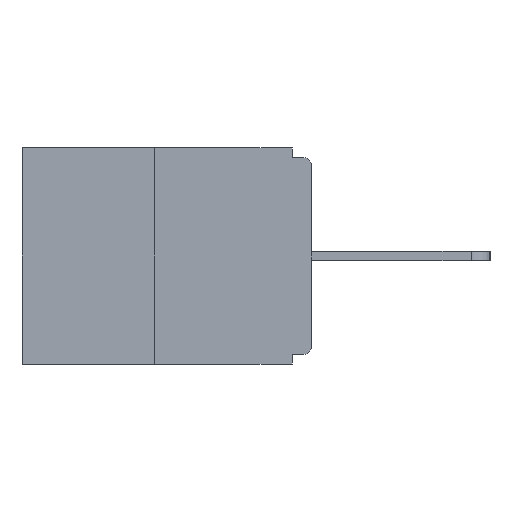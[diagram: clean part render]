
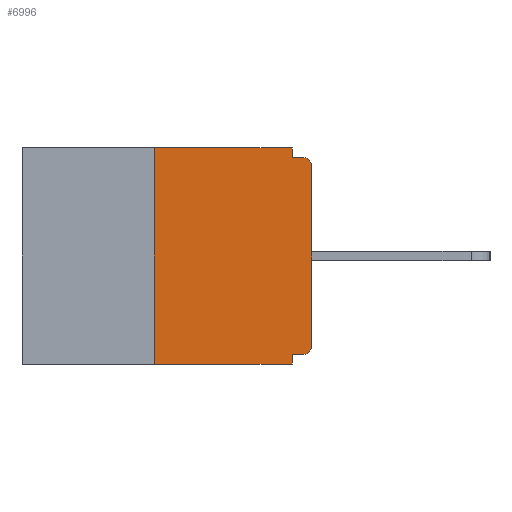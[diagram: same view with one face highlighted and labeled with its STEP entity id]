
A CAD part, left-side view. The second image highlights one B-rep face of the part: STEP entity #6996.
In plain terms, the highlighted planar face has unit normal (-1, 0, 0).
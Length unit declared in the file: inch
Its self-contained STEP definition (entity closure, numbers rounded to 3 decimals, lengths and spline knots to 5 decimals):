
#20 = VERTEX_POINT ( 'NONE', #14427 ) ;
#445 = DIRECTION ( 'NONE',  ( 1., 0., 0. ) ) ;
#558 = DIRECTION ( 'NONE',  ( 0., 0., -1. ) ) ;
#756 = EDGE_CURVE ( 'NONE', #16424, #20, #15112, .T. ) ;
#812 = VECTOR ( 'NONE', #18427, 39.37008 ) ;
#817 = FACE_OUTER_BOUND ( 'NONE', #5721, .T. ) ;
#1799 = CARTESIAN_POINT ( 'NONE',  ( 0., 0.031, -0.015 ) ) ;
#2347 = CARTESIAN_POINT ( 'NONE',  ( 0., 0.25, -0.343 ) ) ;
#2407 = DIRECTION ( 'NONE',  ( 0., -1., 0. ) ) ;
#2481 = DIRECTION ( 'NONE',  ( -1., 0., 0. ) ) ;
#3630 = VERTEX_POINT ( 'NONE', #19188 ) ;
#3812 = VECTOR ( 'NONE', #23161, 39.37008 ) ;
#4531 = VECTOR ( 'NONE', #9648, 39.37008 ) ;
#4666 = LINE ( 'NONE', #21552, #6820 ) ;
#4781 = DIRECTION ( 'NONE',  ( 0., 1., 0. ) ) ;
#5007 = CARTESIAN_POINT ( 'NONE',  ( 0., 0.031, 0. ) ) ;
#5657 = EDGE_CURVE ( 'NONE', #18323, #8845, #22203, .T. ) ;
#5721 = EDGE_LOOP ( 'NONE', ( #11944, #8549, #6640, #10354, #20178, #6721, #15885, #15795, #6546, #6243 ) ) ;
#6027 = AXIS2_PLACEMENT_3D ( 'NONE', #13795, #445, #558 ) ;
#6057 = LINE ( 'NONE', #11752, #11845 ) ;
#6243 = ORIENTED_EDGE ( 'NONE', *, *, #13133, .F. ) ;
#6263 = DIRECTION ( 'NONE',  ( 0., 0., -1. ) ) ;
#6546 = ORIENTED_EDGE ( 'NONE', *, *, #17191, .F. ) ;
#6640 = ORIENTED_EDGE ( 'NONE', *, *, #12163, .T. ) ;
#6721 = ORIENTED_EDGE ( 'NONE', *, *, #5657, .T. ) ;
#6820 = VECTOR ( 'NONE', #4781, 39.37008 ) ;
#6838 = VERTEX_POINT ( 'NONE', #1799 ) ;
#6942 = VERTEX_POINT ( 'NONE', #17453 ) ;
#6996 = ADVANCED_FACE ( 'NONE', ( #817 ), #7982, .F. ) ;
#7363 = VECTOR ( 'NONE', #10056, 39.37008 ) ;
#7982 = PLANE ( 'NONE',  #6027 ) ;
#8549 = ORIENTED_EDGE ( 'NONE', *, *, #756, .F. ) ;
#8809 = CARTESIAN_POINT ( 'NONE',  ( 0., 0., -0.313 ) ) ;
#8845 = VERTEX_POINT ( 'NONE', #8809 ) ;
#9278 = CIRCLE ( 'NONE', #10869, 0.015 ) ;
#9288 = LINE ( 'NONE', #16915, #4531 ) ;
#9648 = DIRECTION ( 'NONE',  ( 0., 0., -1. ) ) ;
#9789 = CARTESIAN_POINT ( 'NONE',  ( 0., 0.25, 0. ) ) ;
#10056 = DIRECTION ( 'NONE',  ( 0., 0., 1. ) ) ;
#10258 = DIRECTION ( 'NONE',  ( 0., 0., -1. ) ) ;
#10354 = ORIENTED_EDGE ( 'NONE', *, *, #17953, .F. ) ;
#10702 = CARTESIAN_POINT ( 'NONE',  ( 0., 0.031, -0.343 ) ) ;
#10869 = AXIS2_PLACEMENT_3D ( 'NONE', #19978, #23193, #10258 ) ;
#11499 = CARTESIAN_POINT ( 'NONE',  ( 0., 0., 0. ) ) ;
#11752 = CARTESIAN_POINT ( 'NONE',  ( 0., 0., -0.015 ) ) ;
#11845 = VECTOR ( 'NONE', #2407, 39.37008 ) ;
#11944 = ORIENTED_EDGE ( 'NONE', *, *, #14705, .F. ) ;
#12163 = EDGE_CURVE ( 'NONE', #16424, #15268, #12847, .T. ) ;
#12847 = LINE ( 'NONE', #14769, #812 ) ;
#13133 = EDGE_CURVE ( 'NONE', #16495, #6838, #17632, .T. ) ;
#13151 = CARTESIAN_POINT ( 'NONE',  ( 0., 0.015, -0.015 ) ) ;
#13405 = LINE ( 'NONE', #15346, #19123 ) ;
#13795 = CARTESIAN_POINT ( 'NONE',  ( 0., 0.46, 0. ) ) ;
#14161 = VECTOR ( 'NONE', #22584, 39.37008 ) ;
#14387 = EDGE_CURVE ( 'NONE', #18323, #6942, #4666, .T. ) ;
#14427 = CARTESIAN_POINT ( 'NONE',  ( 0., 0.25, 0. ) ) ;
#14705 = EDGE_CURVE ( 'NONE', #20, #16495, #13405, .T. ) ;
#14769 = CARTESIAN_POINT ( 'NONE',  ( 0., 0.46, -0.343 ) ) ;
#14790 = EDGE_CURVE ( 'NONE', #3630, #22030, #9278, .T. ) ;
#15112 = LINE ( 'NONE', #9789, #14161 ) ;
#15154 = AXIS2_PLACEMENT_3D ( 'NONE', #20842, #2481, #6263 ) ;
#15268 = VERTEX_POINT ( 'NONE', #10702 ) ;
#15346 = CARTESIAN_POINT ( 'NONE',  ( 0., 0.46, 0. ) ) ;
#15795 = ORIENTED_EDGE ( 'NONE', *, *, #14790, .T. ) ;
#15885 = ORIENTED_EDGE ( 'NONE', *, *, #22948, .T. ) ;
#16424 = VERTEX_POINT ( 'NONE', #2347 ) ;
#16495 = VERTEX_POINT ( 'NONE', #21557 ) ;
#16915 = CARTESIAN_POINT ( 'NONE',  ( 0., 0.031, -0.343 ) ) ;
#17191 = EDGE_CURVE ( 'NONE', #6838, #22030, #6057, .T. ) ;
#17453 = CARTESIAN_POINT ( 'NONE',  ( 0., 0.031, -0.328 ) ) ;
#17550 = DIRECTION ( 'NONE',  ( 0., -1., 0. ) ) ;
#17632 = LINE ( 'NONE', #5007, #3812 ) ;
#17953 = EDGE_CURVE ( 'NONE', #6942, #15268, #9288, .T. ) ;
#18323 = VERTEX_POINT ( 'NONE', #18449 ) ;
#18427 = DIRECTION ( 'NONE',  ( 0., -1., 0. ) ) ;
#18449 = CARTESIAN_POINT ( 'NONE',  ( 0., 0.015, -0.328 ) ) ;
#19123 = VECTOR ( 'NONE', #17550, 39.37008 ) ;
#19188 = CARTESIAN_POINT ( 'NONE',  ( 0., 0., -0.03 ) ) ;
#19978 = CARTESIAN_POINT ( 'NONE',  ( 0., 0.015, -0.03 ) ) ;
#20178 = ORIENTED_EDGE ( 'NONE', *, *, #14387, .F. ) ;
#20739 = LINE ( 'NONE', #11499, #7363 ) ;
#20842 = CARTESIAN_POINT ( 'NONE',  ( 0., 0.015, -0.313 ) ) ;
#21552 = CARTESIAN_POINT ( 'NONE',  ( 0., 0., -0.328 ) ) ;
#21557 = CARTESIAN_POINT ( 'NONE',  ( 0., 0.031, 0. ) ) ;
#22030 = VERTEX_POINT ( 'NONE', #13151 ) ;
#22203 = CIRCLE ( 'NONE', #15154, 0.015 ) ;
#22584 = DIRECTION ( 'NONE',  ( 0., 0., 1. ) ) ;
#22948 = EDGE_CURVE ( 'NONE', #8845, #3630, #20739, .T. ) ;
#23161 = DIRECTION ( 'NONE',  ( 0., 0., -1. ) ) ;
#23193 = DIRECTION ( 'NONE',  ( -1., 0., 0. ) ) ;
